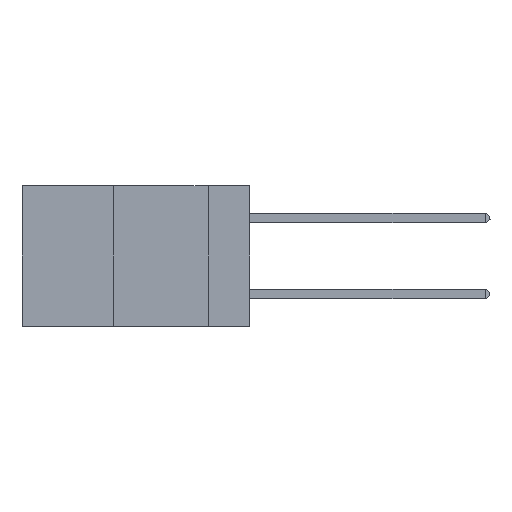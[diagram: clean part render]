
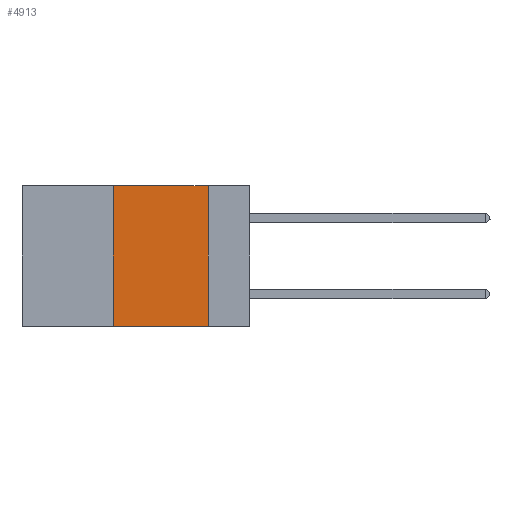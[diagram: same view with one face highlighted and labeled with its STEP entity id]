
A CAD part, left-side view. The second image highlights one B-rep face of the part: STEP entity #4913.
In plain terms, the highlighted planar face has unit normal (-1, 0, 0).
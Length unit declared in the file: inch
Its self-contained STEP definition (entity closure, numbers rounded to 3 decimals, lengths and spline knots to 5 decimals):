
#941 = CARTESIAN_POINT ( 'NONE',  ( 0., 0.11, 0. ) ) ;
#1045 = CARTESIAN_POINT ( 'NONE',  ( 0., 0.11, -0.37 ) ) ;
#2968 = CARTESIAN_POINT ( 'NONE',  ( 0., 0.6, -0.37 ) ) ;
#3336 = EDGE_CURVE ( 'NONE', #11866, #10051, #17665, .T. ) ;
#3463 = DIRECTION ( 'NONE',  ( 0., 0., -1. ) ) ;
#3579 = VERTEX_POINT ( 'NONE', #16984 ) ;
#4038 = DIRECTION ( 'NONE',  ( 0., 0., -1. ) ) ;
#4121 = DIRECTION ( 'NONE',  ( 0., 0., 1. ) ) ;
#4698 = EDGE_CURVE ( 'NONE', #3579, #11866, #14750, .T. ) ;
#4774 = EDGE_CURVE ( 'NONE', #14447, #10051, #14843, .T. ) ;
#4913 = ADVANCED_FACE ( 'NONE', ( #18537 ), #15435, .F. ) ;
#5783 = DIRECTION ( 'NONE',  ( 0., -1., 0. ) ) ;
#7124 = EDGE_LOOP ( 'NONE', ( #8950, #9180, #10225, #9508 ) ) ;
#8950 = ORIENTED_EDGE ( 'NONE', *, *, #3336, .F. ) ;
#9180 = ORIENTED_EDGE ( 'NONE', *, *, #4698, .F. ) ;
#9508 = ORIENTED_EDGE ( 'NONE', *, *, #4774, .T. ) ;
#9576 = DIRECTION ( 'NONE',  ( 1., 0., 0. ) ) ;
#10051 = VERTEX_POINT ( 'NONE', #1045 ) ;
#10225 = ORIENTED_EDGE ( 'NONE', *, *, #12274, .F. ) ;
#11065 = CARTESIAN_POINT ( 'NONE',  ( 0., 0.6, 0. ) ) ;
#11362 = CARTESIAN_POINT ( 'NONE',  ( 0., 0.6, 0. ) ) ;
#11866 = VERTEX_POINT ( 'NONE', #15689 ) ;
#12274 = EDGE_CURVE ( 'NONE', #14447, #3579, #19125, .T. ) ;
#12476 = CARTESIAN_POINT ( 'NONE',  ( 0., 0.36, -0.37 ) ) ;
#13580 = DIRECTION ( 'NONE',  ( 0., -1., 0. ) ) ;
#14418 = VECTOR ( 'NONE', #5783, 39.37008 ) ;
#14447 = VERTEX_POINT ( 'NONE', #12476 ) ;
#14750 = LINE ( 'NONE', #11362, #14418 ) ;
#14843 = LINE ( 'NONE', #2968, #18142 ) ;
#15435 = PLANE ( 'NONE',  #16911 ) ;
#15689 = CARTESIAN_POINT ( 'NONE',  ( 0., 0.11, 0. ) ) ;
#15735 = CARTESIAN_POINT ( 'NONE',  ( 0., 0.36, 0. ) ) ;
#16242 = VECTOR ( 'NONE', #4038, 39.37008 ) ;
#16440 = VECTOR ( 'NONE', #4121, 39.37008 ) ;
#16911 = AXIS2_PLACEMENT_3D ( 'NONE', #11065, #9576, #3463 ) ;
#16984 = CARTESIAN_POINT ( 'NONE',  ( 0., 0.36, 0. ) ) ;
#17665 = LINE ( 'NONE', #941, #16242 ) ;
#18142 = VECTOR ( 'NONE', #13580, 39.37008 ) ;
#18537 = FACE_OUTER_BOUND ( 'NONE', #7124, .T. ) ;
#19125 = LINE ( 'NONE', #15735, #16440 ) ;
